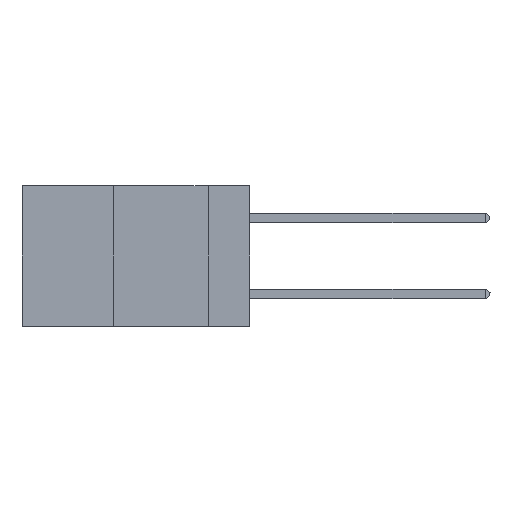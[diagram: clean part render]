
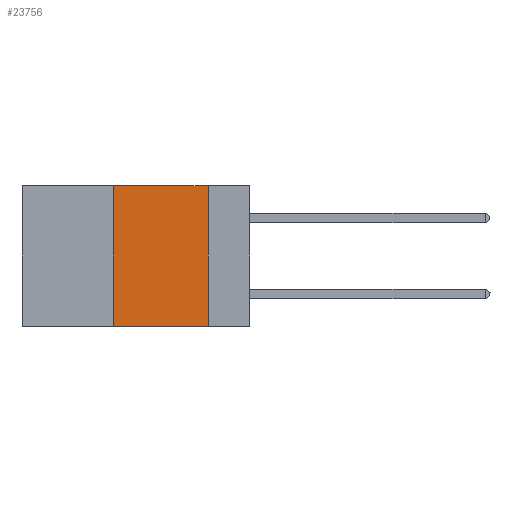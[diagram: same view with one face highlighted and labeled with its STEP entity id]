
A CAD part, left-side view. The second image highlights one B-rep face of the part: STEP entity #23756.
In plain terms, the highlighted planar face has unit normal (-1, 0, 0).
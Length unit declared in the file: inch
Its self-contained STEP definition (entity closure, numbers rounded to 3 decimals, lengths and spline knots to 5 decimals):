
#1883 = CARTESIAN_POINT ( 'NONE',  ( 0., 0.36, -0.37 ) ) ;
#5533 = DIRECTION ( 'NONE',  ( 0., 0., -1. ) ) ;
#6094 = LINE ( 'NONE', #24384, #14530 ) ;
#6410 = FACE_OUTER_BOUND ( 'NONE', #22555, .T. ) ;
#7602 = VERTEX_POINT ( 'NONE', #12681 ) ;
#7607 = VECTOR ( 'NONE', #18651, 39.37008 ) ;
#9402 = AXIS2_PLACEMENT_3D ( 'NONE', #16219, #26812, #5533 ) ;
#10235 = ORIENTED_EDGE ( 'NONE', *, *, #26961, .F. ) ;
#12282 = CARTESIAN_POINT ( 'NONE',  ( 0., 0.6, -0.37 ) ) ;
#12681 = CARTESIAN_POINT ( 'NONE',  ( 0., 0.11, 0. ) ) ;
#14530 = VECTOR ( 'NONE', #24693, 39.37008 ) ;
#16171 = CARTESIAN_POINT ( 'NONE',  ( 0., 0.11, -0.37 ) ) ;
#16219 = CARTESIAN_POINT ( 'NONE',  ( 0., 0.6, 0. ) ) ;
#17033 = ORIENTED_EDGE ( 'NONE', *, *, #25729, .T. ) ;
#17193 = LINE ( 'NONE', #39263, #7607 ) ;
#18602 = LINE ( 'NONE', #12282, #35864 ) ;
#18651 = DIRECTION ( 'NONE',  ( 0., -1., 0. ) ) ;
#22227 = EDGE_CURVE ( 'NONE', #39236, #7602, #17193, .T. ) ;
#22555 = EDGE_LOOP ( 'NONE', ( #10235, #25264, #43476, #17033 ) ) ;
#23330 = VECTOR ( 'NONE', #30276, 39.37008 ) ;
#23756 = ADVANCED_FACE ( 'NONE', ( #6410 ), #30122, .F. ) ;
#24384 = CARTESIAN_POINT ( 'NONE',  ( 0., 0.11, 0. ) ) ;
#24693 = DIRECTION ( 'NONE',  ( 0., 0., -1. ) ) ;
#25264 = ORIENTED_EDGE ( 'NONE', *, *, #22227, .F. ) ;
#25729 = EDGE_CURVE ( 'NONE', #36676, #29704, #18602, .T. ) ;
#26812 = DIRECTION ( 'NONE',  ( 1., 0., 0. ) ) ;
#26961 = EDGE_CURVE ( 'NONE', #7602, #29704, #6094, .T. ) ;
#28943 = CARTESIAN_POINT ( 'NONE',  ( 0., 0.36, 0. ) ) ;
#29704 = VERTEX_POINT ( 'NONE', #16171 ) ;
#30122 = PLANE ( 'NONE',  #9402 ) ;
#30276 = DIRECTION ( 'NONE',  ( 0., 0., 1. ) ) ;
#32487 = LINE ( 'NONE', #43873, #23330 ) ;
#35864 = VECTOR ( 'NONE', #40088, 39.37008 ) ;
#36676 = VERTEX_POINT ( 'NONE', #1883 ) ;
#39236 = VERTEX_POINT ( 'NONE', #28943 ) ;
#39263 = CARTESIAN_POINT ( 'NONE',  ( 0., 0.6, 0. ) ) ;
#39473 = EDGE_CURVE ( 'NONE', #36676, #39236, #32487, .T. ) ;
#40088 = DIRECTION ( 'NONE',  ( 0., -1., 0. ) ) ;
#43476 = ORIENTED_EDGE ( 'NONE', *, *, #39473, .F. ) ;
#43873 = CARTESIAN_POINT ( 'NONE',  ( 0., 0.36, 0. ) ) ;
